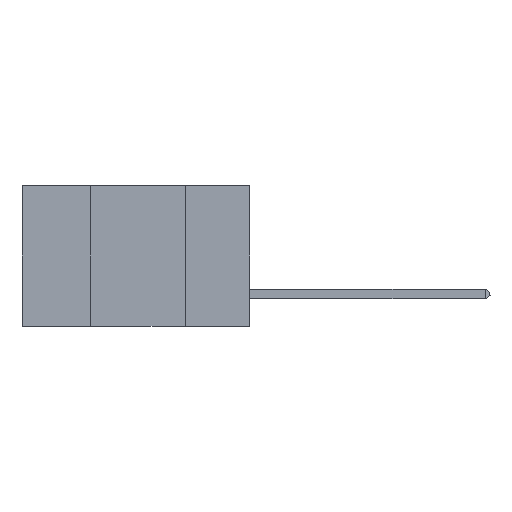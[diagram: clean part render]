
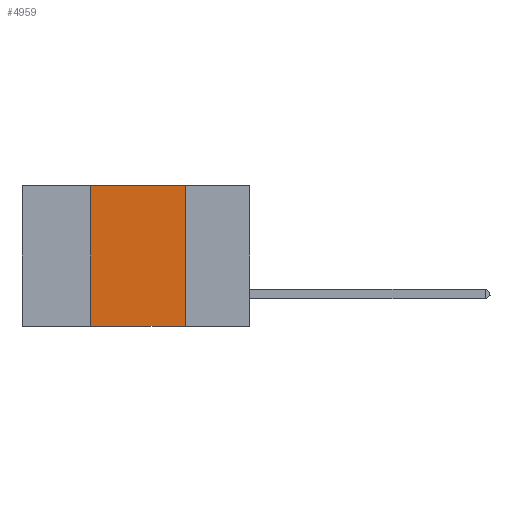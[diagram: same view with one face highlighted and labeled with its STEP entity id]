
A CAD part, left-side view. The second image highlights one B-rep face of the part: STEP entity #4959.
In plain terms, the highlighted planar face has unit normal (-1, 0, 0).
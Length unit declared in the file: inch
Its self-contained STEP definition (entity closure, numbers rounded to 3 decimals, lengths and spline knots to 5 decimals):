
#212 = AXIS2_PLACEMENT_3D ( 'NONE', #7582, #7622, #3943 ) ;
#392 = ORIENTED_EDGE ( 'NONE', *, *, #6207, .F. ) ;
#540 = CARTESIAN_POINT ( 'NONE',  ( 0., 0.17, 0. ) ) ;
#654 = CARTESIAN_POINT ( 'NONE',  ( 0., 0.6, -0.37 ) ) ;
#833 = EDGE_LOOP ( 'NONE', ( #392, #5659, #6508, #7863 ) ) ;
#963 = DIRECTION ( 'NONE',  ( 0., 0., 1. ) ) ;
#974 = VERTEX_POINT ( 'NONE', #540 ) ;
#1936 = LINE ( 'NONE', #8807, #7246 ) ;
#2823 = CARTESIAN_POINT ( 'NONE',  ( 0., 0.17, -0.37 ) ) ;
#3943 = DIRECTION ( 'NONE',  ( 0., 0., -1. ) ) ;
#4052 = PLANE ( 'NONE',  #212 ) ;
#4117 = DIRECTION ( 'NONE',  ( 0., -1., 0. ) ) ;
#4233 = DIRECTION ( 'NONE',  ( 0., -1., 0. ) ) ;
#4959 = ADVANCED_FACE ( 'NONE', ( #11022 ), #4052, .F. ) ;
#5227 = CARTESIAN_POINT ( 'NONE',  ( 0., 0.6, 0. ) ) ;
#5659 = ORIENTED_EDGE ( 'NONE', *, *, #14266, .F. ) ;
#5691 = VECTOR ( 'NONE', #4117, 39.37008 ) ;
#6023 = CARTESIAN_POINT ( 'NONE',  ( 0., 0.42, -0.37 ) ) ;
#6207 = EDGE_CURVE ( 'NONE', #974, #8132, #1936, .T. ) ;
#6508 = ORIENTED_EDGE ( 'NONE', *, *, #10983, .F. ) ;
#7246 = VECTOR ( 'NONE', #10411, 39.37008 ) ;
#7582 = CARTESIAN_POINT ( 'NONE',  ( 0., 0.6, 0. ) ) ;
#7622 = DIRECTION ( 'NONE',  ( 1., 0., 0. ) ) ;
#7863 = ORIENTED_EDGE ( 'NONE', *, *, #14492, .T. ) ;
#8132 = VERTEX_POINT ( 'NONE', #2823 ) ;
#8759 = VERTEX_POINT ( 'NONE', #16232 ) ;
#8807 = CARTESIAN_POINT ( 'NONE',  ( 0., 0.17, 0. ) ) ;
#9018 = LINE ( 'NONE', #5227, #5691 ) ;
#10411 = DIRECTION ( 'NONE',  ( 0., 0., -1. ) ) ;
#10983 = EDGE_CURVE ( 'NONE', #14128, #8759, #12494, .T. ) ;
#11022 = FACE_OUTER_BOUND ( 'NONE', #833, .T. ) ;
#12494 = LINE ( 'NONE', #13481, #14860 ) ;
#13481 = CARTESIAN_POINT ( 'NONE',  ( 0., 0.42, 0. ) ) ;
#14117 = LINE ( 'NONE', #654, #15489 ) ;
#14128 = VERTEX_POINT ( 'NONE', #6023 ) ;
#14266 = EDGE_CURVE ( 'NONE', #8759, #974, #9018, .T. ) ;
#14492 = EDGE_CURVE ( 'NONE', #14128, #8132, #14117, .T. ) ;
#14860 = VECTOR ( 'NONE', #963, 39.37008 ) ;
#15489 = VECTOR ( 'NONE', #4233, 39.37008 ) ;
#16232 = CARTESIAN_POINT ( 'NONE',  ( 0., 0.42, 0. ) ) ;
